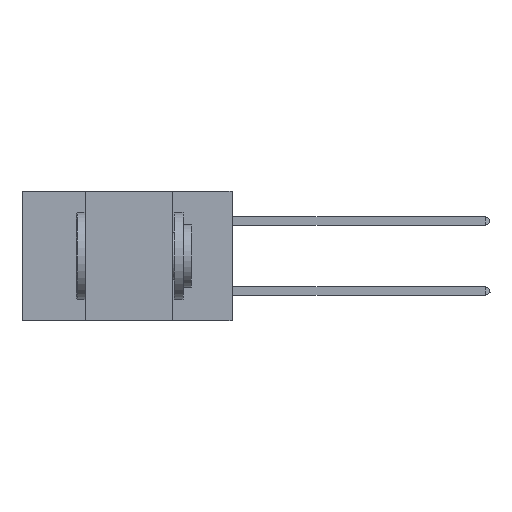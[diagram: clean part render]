
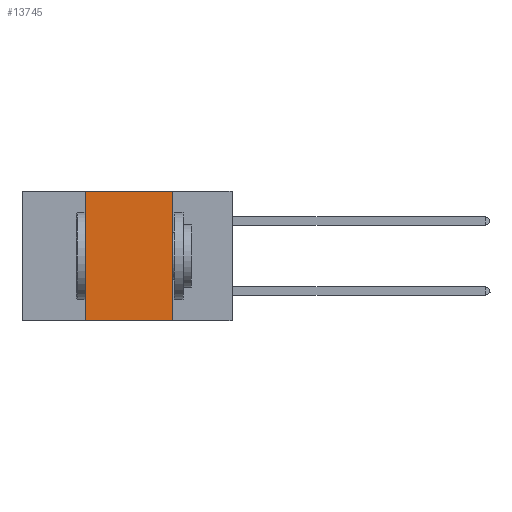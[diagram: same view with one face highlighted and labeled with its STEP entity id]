
A CAD part, left-side view. The second image highlights one B-rep face of the part: STEP entity #13745.
In plain terms, the highlighted planar face has unit normal (-1, 0, 0).
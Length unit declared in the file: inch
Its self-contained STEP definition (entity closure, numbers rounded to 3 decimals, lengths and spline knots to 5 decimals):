
#1292 = EDGE_CURVE ( 'NONE', #24636, #20478, #16067, .T. ) ;
#2557 = VECTOR ( 'NONE', #16483, 39.37008 ) ;
#2919 = CARTESIAN_POINT ( 'NONE',  ( 0., 0.42, 0. ) ) ;
#3075 = PLANE ( 'NONE',  #4726 ) ;
#3230 = VECTOR ( 'NONE', #30782, 39.37008 ) ;
#3630 = EDGE_CURVE ( 'NONE', #24636, #12849, #12077, .T. ) ;
#3824 = DIRECTION ( 'NONE',  ( 1., 0., 0. ) ) ;
#4395 = ORIENTED_EDGE ( 'NONE', *, *, #1292, .F. ) ;
#4654 = CARTESIAN_POINT ( 'NONE',  ( 0., 0.42, -0.37 ) ) ;
#4726 = AXIS2_PLACEMENT_3D ( 'NONE', #25739, #3824, #24345 ) ;
#4831 = VERTEX_POINT ( 'NONE', #6575 ) ;
#6425 = ORIENTED_EDGE ( 'NONE', *, *, #3630, .T. ) ;
#6575 = CARTESIAN_POINT ( 'NONE',  ( 0., 0.17, 0. ) ) ;
#7675 = CARTESIAN_POINT ( 'NONE',  ( 0., 0.6, -0.37 ) ) ;
#11197 = EDGE_CURVE ( 'NONE', #4831, #12849, #13755, .T. ) ;
#11285 = DIRECTION ( 'NONE',  ( 0., -1., 0. ) ) ;
#11420 = EDGE_LOOP ( 'NONE', ( #27809, #30249, #4395, #6425 ) ) ;
#12077 = LINE ( 'NONE', #7675, #3230 ) ;
#12849 = VERTEX_POINT ( 'NONE', #26745 ) ;
#13509 = LINE ( 'NONE', #13625, #21946 ) ;
#13625 = CARTESIAN_POINT ( 'NONE',  ( 0., 0.6, 0. ) ) ;
#13745 = ADVANCED_FACE ( 'NONE', ( #20782 ), #3075, .F. ) ;
#13755 = LINE ( 'NONE', #21770, #2557 ) ;
#16067 = LINE ( 'NONE', #30479, #26110 ) ;
#16483 = DIRECTION ( 'NONE',  ( 0., 0., -1. ) ) ;
#17873 = DIRECTION ( 'NONE',  ( 0., 0., 1. ) ) ;
#20478 = VERTEX_POINT ( 'NONE', #2919 ) ;
#20782 = FACE_OUTER_BOUND ( 'NONE', #11420, .T. ) ;
#21770 = CARTESIAN_POINT ( 'NONE',  ( 0., 0.17, 0. ) ) ;
#21946 = VECTOR ( 'NONE', #11285, 39.37008 ) ;
#24345 = DIRECTION ( 'NONE',  ( 0., 0., -1. ) ) ;
#24636 = VERTEX_POINT ( 'NONE', #4654 ) ;
#25739 = CARTESIAN_POINT ( 'NONE',  ( 0., 0.6, 0. ) ) ;
#26110 = VECTOR ( 'NONE', #17873, 39.37008 ) ;
#26607 = EDGE_CURVE ( 'NONE', #20478, #4831, #13509, .T. ) ;
#26745 = CARTESIAN_POINT ( 'NONE',  ( 0., 0.17, -0.37 ) ) ;
#27809 = ORIENTED_EDGE ( 'NONE', *, *, #11197, .F. ) ;
#30249 = ORIENTED_EDGE ( 'NONE', *, *, #26607, .F. ) ;
#30479 = CARTESIAN_POINT ( 'NONE',  ( 0., 0.42, 0. ) ) ;
#30782 = DIRECTION ( 'NONE',  ( 0., -1., 0. ) ) ;
